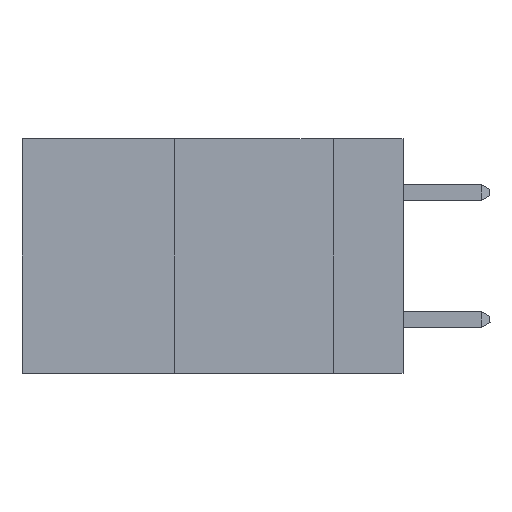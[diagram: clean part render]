
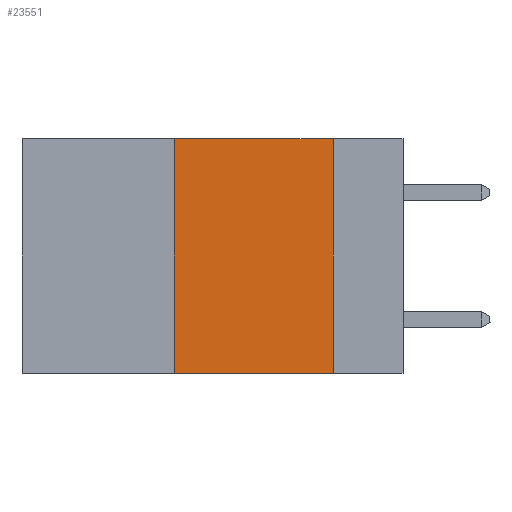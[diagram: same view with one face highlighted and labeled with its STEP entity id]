
A CAD part, left-side view. The second image highlights one B-rep face of the part: STEP entity #23551.
In plain terms, the highlighted planar face has unit normal (-1, 0, 0).
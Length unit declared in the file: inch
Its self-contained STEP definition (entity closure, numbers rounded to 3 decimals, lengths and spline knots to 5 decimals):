
#409 = VECTOR ( 'NONE', #23477, 39.37008 ) ;
#919 = LINE ( 'NONE', #8375, #1604 ) ;
#1604 = VECTOR ( 'NONE', #10533, 39.37008 ) ;
#2474 = VECTOR ( 'NONE', #20077, 39.37008 ) ;
#2598 = VERTEX_POINT ( 'NONE', #7832 ) ;
#4063 = VERTEX_POINT ( 'NONE', #14321 ) ;
#5282 = ORIENTED_EDGE ( 'NONE', *, *, #26497, .T. ) ;
#5774 = ORIENTED_EDGE ( 'NONE', *, *, #19783, .F. ) ;
#7832 = CARTESIAN_POINT ( 'NONE',  ( 0., 0.11, 0. ) ) ;
#8243 = CARTESIAN_POINT ( 'NONE',  ( 0., 0.11, 0. ) ) ;
#8375 = CARTESIAN_POINT ( 'NONE',  ( 0., 0.36, 0. ) ) ;
#9584 = LINE ( 'NONE', #11599, #2474 ) ;
#9804 = EDGE_LOOP ( 'NONE', ( #11760, #5774, #11399, #5282 ) ) ;
#10533 = DIRECTION ( 'NONE',  ( 0., 0., 1. ) ) ;
#11271 = FACE_OUTER_BOUND ( 'NONE', #9804, .T. ) ;
#11399 = ORIENTED_EDGE ( 'NONE', *, *, #21128, .F. ) ;
#11599 = CARTESIAN_POINT ( 'NONE',  ( 0., 0.6, -0.37 ) ) ;
#11760 = ORIENTED_EDGE ( 'NONE', *, *, #19311, .F. ) ;
#12523 = LINE ( 'NONE', #8243, #409 ) ;
#13872 = DIRECTION ( 'NONE',  ( 1., 0., 0. ) ) ;
#14321 = CARTESIAN_POINT ( 'NONE',  ( 0., 0.36, 0. ) ) ;
#15441 = VERTEX_POINT ( 'NONE', #25849 ) ;
#18063 = DIRECTION ( 'NONE',  ( 0., -1., 0. ) ) ;
#18153 = CARTESIAN_POINT ( 'NONE',  ( 0., 0.6, 0. ) ) ;
#19311 = EDGE_CURVE ( 'NONE', #2598, #15441, #12523, .T. ) ;
#19473 = VERTEX_POINT ( 'NONE', #23745 ) ;
#19783 = EDGE_CURVE ( 'NONE', #4063, #2598, #20817, .T. ) ;
#20077 = DIRECTION ( 'NONE',  ( 0., -1., 0. ) ) ;
#20709 = CARTESIAN_POINT ( 'NONE',  ( 0., 0.6, 0. ) ) ;
#20817 = LINE ( 'NONE', #18153, #24825 ) ;
#21128 = EDGE_CURVE ( 'NONE', #19473, #4063, #919, .T. ) ;
#22492 = PLANE ( 'NONE',  #27032 ) ;
#22582 = DIRECTION ( 'NONE',  ( 0., 0., -1. ) ) ;
#23477 = DIRECTION ( 'NONE',  ( 0., 0., -1. ) ) ;
#23551 = ADVANCED_FACE ( 'NONE', ( #11271 ), #22492, .F. ) ;
#23745 = CARTESIAN_POINT ( 'NONE',  ( 0., 0.36, -0.37 ) ) ;
#24825 = VECTOR ( 'NONE', #18063, 39.37008 ) ;
#25849 = CARTESIAN_POINT ( 'NONE',  ( 0., 0.11, -0.37 ) ) ;
#26497 = EDGE_CURVE ( 'NONE', #19473, #15441, #9584, .T. ) ;
#27032 = AXIS2_PLACEMENT_3D ( 'NONE', #20709, #13872, #22582 ) ;
